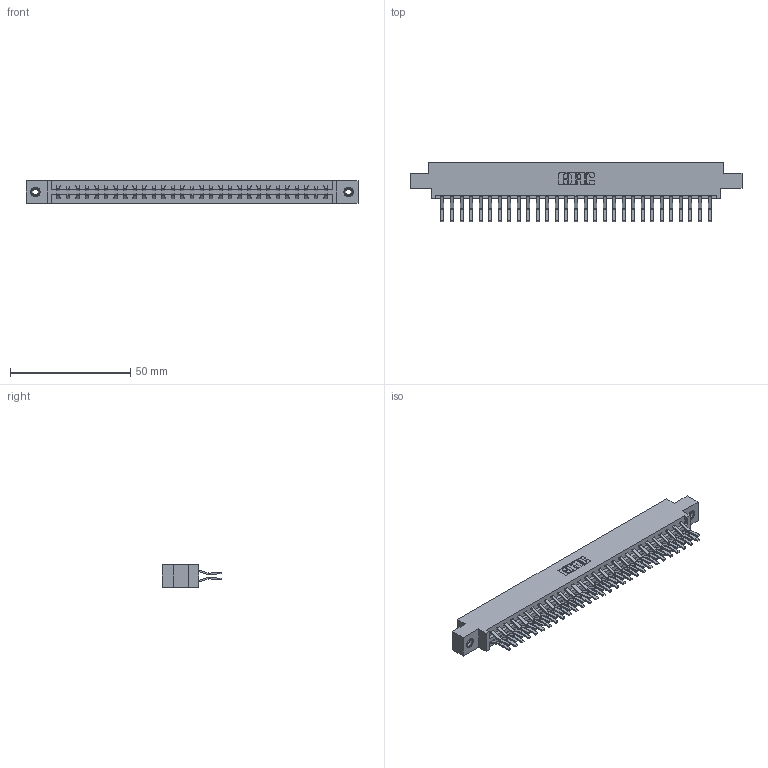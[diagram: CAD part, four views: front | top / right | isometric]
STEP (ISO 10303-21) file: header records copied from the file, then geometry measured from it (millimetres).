
FILE_DESCRIPTION (( 'STEP AP203' ), '1' );
FILE_NAME ('387-058-560-808.STEP', '2019-10-19T10:36:40', ( '' ), ( '' ), 'SwSTEP 2.0', 'SolidWorks 2016', '' );
FILE_SCHEMA (( 'CONFIG_CONTROL_DESIGN' ));
Length unit declared in the file: inch
Products named in the file (4): 345-250-001_345-250-003-102; 337 Part_0.170 Offset - 0.156 Dia-TI; 387-058-560-808; 345-292-001_560 Tail
Assembly tree (61 placements, depth 2):
  387-058-560-808
    337 Part_0.170 Offset - 0.156 Dia-TI
    345-292-001_560 Tail  x58
    345-250-001_345-250-003-102  x2
Bounding box: 137.92 x 24.78 x 9.4 mm (x, y, z)
Volume: 14618.4 mm3; surface area: 17631.9 mm2
Topology: 61 solids, 61 shells, 3426 faces, 10145 edges, 6678 vertices
Faces by surface type: plane 2310, cylinder 1100, cone 12, torus 4
Entity records: 25572 total; most frequent: CARTESIAN_POINT 4301, ORIENTED_EDGE 4230, DIRECTION 3717, EDGE_CURVE 2115, LINE 1963, VECTOR 1963, VERTEX_POINT 1404, AXIS2_PLACEMENT_3D 877
